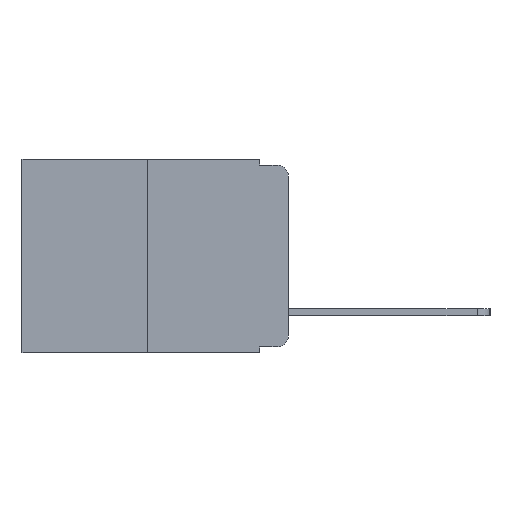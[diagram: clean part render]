
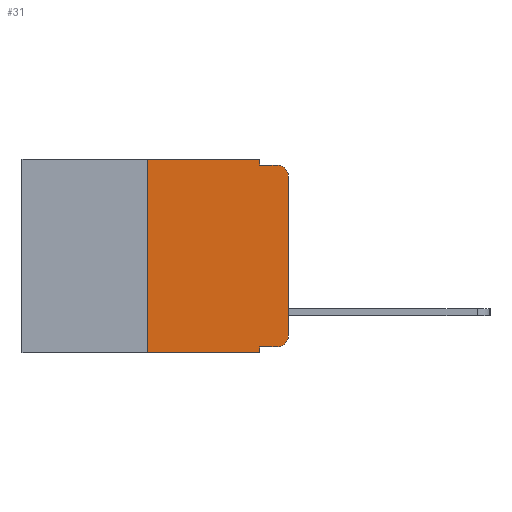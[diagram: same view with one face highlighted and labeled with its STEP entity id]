
A CAD part, left-side view. The second image highlights one B-rep face of the part: STEP entity #31.
In plain terms, the highlighted planar face has unit normal (-1, 0, 0).
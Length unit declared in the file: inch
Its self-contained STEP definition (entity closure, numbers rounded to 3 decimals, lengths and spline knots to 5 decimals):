
#20 = DIRECTION ( 'NONE',  ( 0., -1., 0. ) ) ;
#31 = ADVANCED_FACE ( 'NONE', ( #10631 ), #9899, .F. ) ;
#150 = VERTEX_POINT ( 'NONE', #1293 ) ;
#162 = DIRECTION ( 'NONE',  ( 0., 0., -1. ) ) ;
#432 = DIRECTION ( 'NONE',  ( 1., 0., 0. ) ) ;
#578 = CARTESIAN_POINT ( 'NONE',  ( 0., 0.02, -0.333 ) ) ;
#1248 = VERTEX_POINT ( 'NONE', #5594 ) ;
#1255 = CARTESIAN_POINT ( 'NONE',  ( 0., 0.02, -0.313 ) ) ;
#1293 = CARTESIAN_POINT ( 'NONE',  ( 0., 0.02, -0.01 ) ) ;
#1472 = VERTEX_POINT ( 'NONE', #5093 ) ;
#1913 = EDGE_CURVE ( 'NONE', #4873, #11018, #10811, .T. ) ;
#2026 = CARTESIAN_POINT ( 'NONE',  ( 0., 0.25, -0.343 ) ) ;
#2032 = ORIENTED_EDGE ( 'NONE', *, *, #5898, .T. ) ;
#2251 = DIRECTION ( 'NONE',  ( 0., 0., -1. ) ) ;
#2352 = ORIENTED_EDGE ( 'NONE', *, *, #10161, .T. ) ;
#2603 = DIRECTION ( 'NONE',  ( 0., -1., 0. ) ) ;
#2630 = AXIS2_PLACEMENT_3D ( 'NONE', #9162, #4114, #9938 ) ;
#2962 = CARTESIAN_POINT ( 'NONE',  ( 0., 0.473, -0.343 ) ) ;
#3165 = VECTOR ( 'NONE', #162, 39.37008 ) ;
#3195 = ORIENTED_EDGE ( 'NONE', *, *, #5363, .F. ) ;
#3323 = VERTEX_POINT ( 'NONE', #8918 ) ;
#3521 = AXIS2_PLACEMENT_3D ( 'NONE', #1255, #7464, #2251 ) ;
#3828 = CARTESIAN_POINT ( 'NONE',  ( 0., 0., 0. ) ) ;
#4114 = DIRECTION ( 'NONE',  ( -1., 0., 0. ) ) ;
#4242 = VECTOR ( 'NONE', #2603, 39.37008 ) ;
#4596 = CARTESIAN_POINT ( 'NONE',  ( 0., 0.473, 0. ) ) ;
#4737 = CIRCLE ( 'NONE', #3521, 0.02 ) ;
#4873 = VERTEX_POINT ( 'NONE', #2026 ) ;
#5093 = CARTESIAN_POINT ( 'NONE',  ( 0., 0., -0.313 ) ) ;
#5177 = CARTESIAN_POINT ( 'NONE',  ( 0., 0.051, 0. ) ) ;
#5195 = CARTESIAN_POINT ( 'NONE',  ( 0., 0.051, -0.01 ) ) ;
#5291 = VECTOR ( 'NONE', #6047, 39.37008 ) ;
#5346 = CARTESIAN_POINT ( 'NONE',  ( 0., 0.051, -0.343 ) ) ;
#5363 = EDGE_CURVE ( 'NONE', #1248, #150, #8985, .T. ) ;
#5594 = CARTESIAN_POINT ( 'NONE',  ( 0., 0.051, -0.01 ) ) ;
#5687 = VERTEX_POINT ( 'NONE', #8363 ) ;
#5898 = EDGE_CURVE ( 'NONE', #1472, #3323, #9468, .T. ) ;
#5947 = DIRECTION ( 'NONE',  ( 0., -1., 0. ) ) ;
#6047 = DIRECTION ( 'NONE',  ( 0., -1., 0. ) ) ;
#6183 = EDGE_CURVE ( 'NONE', #4873, #6807, #9363, .T. ) ;
#6235 = LINE ( 'NONE', #10672, #9572 ) ;
#6317 = EDGE_CURVE ( 'NONE', #7905, #11018, #9100, .T. ) ;
#6364 = VECTOR ( 'NONE', #10108, 39.37008 ) ;
#6787 = CARTESIAN_POINT ( 'NONE',  ( 0., 0.25, 0. ) ) ;
#6790 = VECTOR ( 'NONE', #5947, 39.37008 ) ;
#6807 = VERTEX_POINT ( 'NONE', #10600 ) ;
#6852 = EDGE_CURVE ( 'NONE', #6807, #5687, #6235, .T. ) ;
#6938 = EDGE_LOOP ( 'NONE', ( #2032, #2352, #3195, #9955, #10702, #8871, #10337, #9010, #11321, #8783 ) ) ;
#7021 = VECTOR ( 'NONE', #10496, 39.37008 ) ;
#7256 = EDGE_CURVE ( 'NONE', #7905, #9432, #9685, .T. ) ;
#7464 = DIRECTION ( 'NONE',  ( -1., 0., 0. ) ) ;
#7905 = VERTEX_POINT ( 'NONE', #9833 ) ;
#8001 = EDGE_CURVE ( 'NONE', #9432, #1472, #4737, .T. ) ;
#8363 = CARTESIAN_POINT ( 'NONE',  ( 0., 0.051, 0. ) ) ;
#8531 = CARTESIAN_POINT ( 'NONE',  ( 0., 0.051, -0.333 ) ) ;
#8783 = ORIENTED_EDGE ( 'NONE', *, *, #8001, .T. ) ;
#8826 = CIRCLE ( 'NONE', #2630, 0.02 ) ;
#8871 = ORIENTED_EDGE ( 'NONE', *, *, #6183, .F. ) ;
#8918 = CARTESIAN_POINT ( 'NONE',  ( 0., 0., -0.03 ) ) ;
#8985 = LINE ( 'NONE', #5195, #6790 ) ;
#9010 = ORIENTED_EDGE ( 'NONE', *, *, #6317, .F. ) ;
#9100 = LINE ( 'NONE', #5177, #6364 ) ;
#9162 = CARTESIAN_POINT ( 'NONE',  ( 0., 0.02, -0.03 ) ) ;
#9184 = CARTESIAN_POINT ( 'NONE',  ( 0., 0.051, 0. ) ) ;
#9363 = LINE ( 'NONE', #6787, #11162 ) ;
#9432 = VERTEX_POINT ( 'NONE', #578 ) ;
#9468 = LINE ( 'NONE', #3828, #7021 ) ;
#9572 = VECTOR ( 'NONE', #20, 39.37008 ) ;
#9628 = EDGE_CURVE ( 'NONE', #5687, #1248, #9922, .T. ) ;
#9685 = LINE ( 'NONE', #8531, #5291 ) ;
#9697 = DIRECTION ( 'NONE',  ( 0., 0., -1. ) ) ;
#9833 = CARTESIAN_POINT ( 'NONE',  ( 0., 0.051, -0.333 ) ) ;
#9899 = PLANE ( 'NONE',  #10638 ) ;
#9922 = LINE ( 'NONE', #9184, #3165 ) ;
#9938 = DIRECTION ( 'NONE',  ( 0., 0., -1. ) ) ;
#9955 = ORIENTED_EDGE ( 'NONE', *, *, #9628, .F. ) ;
#10011 = DIRECTION ( 'NONE',  ( 0., 0., 1. ) ) ;
#10108 = DIRECTION ( 'NONE',  ( 0., 0., -1. ) ) ;
#10161 = EDGE_CURVE ( 'NONE', #3323, #150, #8826, .T. ) ;
#10337 = ORIENTED_EDGE ( 'NONE', *, *, #1913, .T. ) ;
#10496 = DIRECTION ( 'NONE',  ( 0., 0., 1. ) ) ;
#10600 = CARTESIAN_POINT ( 'NONE',  ( 0., 0.25, 0. ) ) ;
#10631 = FACE_OUTER_BOUND ( 'NONE', #6938, .T. ) ;
#10638 = AXIS2_PLACEMENT_3D ( 'NONE', #4596, #432, #9697 ) ;
#10672 = CARTESIAN_POINT ( 'NONE',  ( 0., 0.473, 0. ) ) ;
#10702 = ORIENTED_EDGE ( 'NONE', *, *, #6852, .F. ) ;
#10811 = LINE ( 'NONE', #2962, #4242 ) ;
#11018 = VERTEX_POINT ( 'NONE', #5346 ) ;
#11162 = VECTOR ( 'NONE', #10011, 39.37008 ) ;
#11321 = ORIENTED_EDGE ( 'NONE', *, *, #7256, .T. ) ;
